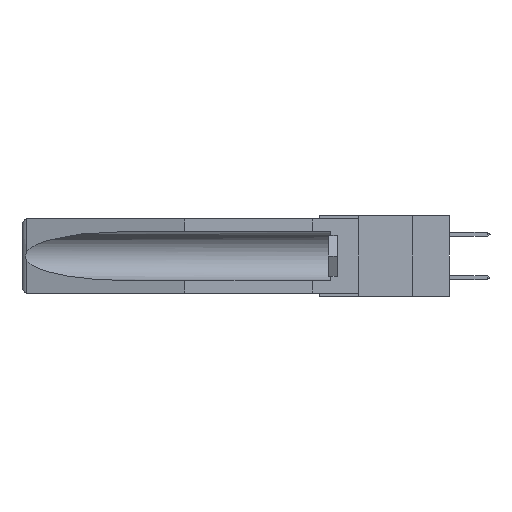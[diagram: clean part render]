
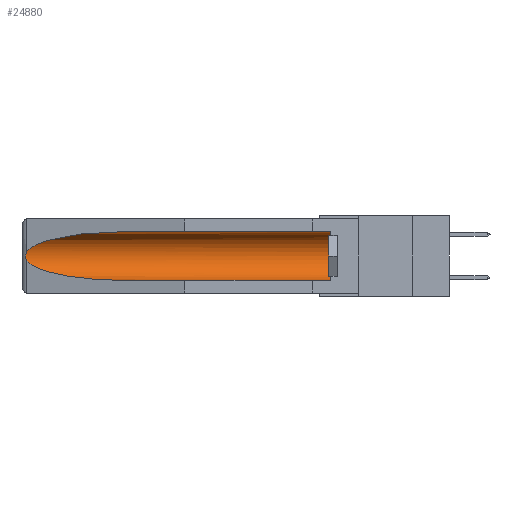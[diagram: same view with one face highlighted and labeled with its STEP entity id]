
A CAD part, left-side view. The second image highlights one B-rep face of the part: STEP entity #24880.
In plain terms, the highlighted cylindrical face has radius 2.857 mm (diameter 5.715 mm), a partial arc.
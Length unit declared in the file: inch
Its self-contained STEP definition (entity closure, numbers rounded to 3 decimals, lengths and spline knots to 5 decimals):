
#214 = DIRECTION ( 'NONE',  ( 0., 1., 0. ) ) ;
#863 = CARTESIAN_POINT ( 'NONE',  ( 0.26537, 1.52718, -0.19328 ) ) ;
#1735 = AXIS2_PLACEMENT_3D ( 'NONE', #17548, #19934, #3326 ) ;
#1859 = EDGE_CURVE ( 'NONE', #19956, #7978, #10673, .T. ) ;
#3016 = CARTESIAN_POINT ( 'NONE',  ( 0.155, 1.07973, -0.059 ) ) ;
#3326 = DIRECTION ( 'NONE',  ( 0., 0., 1. ) ) ;
#3481 = CARTESIAN_POINT ( 'NONE',  ( 0.26537, 1.52718, -0.14972 ) ) ;
#3606 =( BOUNDED_CURVE ( )  B_SPLINE_CURVE ( 3, ( #11257, #11065, #22783, #15631 ),
 .UNSPECIFIED., .F., .F. ) 
 B_SPLINE_CURVE_WITH_KNOTS ( ( 4, 4 ),
 ( 0.1948, 1.5708 ),
 .UNSPECIFIED. ) 
 CURVE ( )  GEOMETRIC_REPRESENTATION_ITEM ( )  RATIONAL_B_SPLINE_CURVE ( ( 1., 0.848, 0.848, 1. ) ) 
 REPRESENTATION_ITEM ( '' )  );
#3780 = EDGE_CURVE ( 'NONE', #7156, #20496, #21490, .T. ) ;
#5236 = EDGE_LOOP ( 'NONE', ( #13361, #5335, #15770, #25116, #20917, #25081 ) ) ;
#5335 = ORIENTED_EDGE ( 'NONE', *, *, #9148, .T. ) ;
#6289 = CARTESIAN_POINT ( 'NONE',  ( 0.2675, 1.53308, -0.17534 ) ) ;
#7156 = VERTEX_POINT ( 'NONE', #22638 ) ;
#7978 = VERTEX_POINT ( 'NONE', #10815 ) ;
#8559 = CARTESIAN_POINT ( 'NONE',  ( 0.26537, 1.52718, -0.14972 ) ) ;
#8656 = CARTESIAN_POINT ( 'NONE',  ( 0.2673, 1.5327, -0.16383 ) ) ;
#9148 = EDGE_CURVE ( 'NONE', #20496, #27413, #15591, .T. ) ;
#9600 = VERTEX_POINT ( 'NONE', #24937 ) ;
#10149 = CARTESIAN_POINT ( 'NONE',  ( 0.155, -0.30754, -0.1715 ) ) ;
#10673 = CIRCLE ( 'NONE', #1735, 0.1125 ) ;
#10815 = CARTESIAN_POINT ( 'NONE',  ( 0.155, 0.126, -0.059 ) ) ;
#11011 = CARTESIAN_POINT ( 'NONE',  ( 0.26537, 1.52718, -0.19328 ) ) ;
#11060 = CARTESIAN_POINT ( 'NONE',  ( 0.26597, 1.5296, -0.19026 ) ) ;
#11065 = CARTESIAN_POINT ( 'NONE',  ( 0.25451, 1.48313, -0.24835 ) ) ;
#11257 = CARTESIAN_POINT ( 'NONE',  ( 0.26537, 1.52718, -0.19328 ) ) ;
#13358 = CARTESIAN_POINT ( 'NONE',  ( 0.26654, 1.53092, -0.15636 ) ) ;
#13361 = ORIENTED_EDGE ( 'NONE', *, *, #3780, .T. ) ;
#14021 = DIRECTION ( 'NONE',  ( 0., 1., 0. ) ) ;
#14847 = LINE ( 'NONE', #25965, #16313 ) ;
#15588 = CARTESIAN_POINT ( 'NONE',  ( 0.155, 0.126, -0.284 ) ) ;
#15591 = B_SPLINE_CURVE_WITH_KNOTS ( 'NONE', 3,
 ( #8559, #27561, #13358, #8656, #18232, #6289, #24556, #26954, #11060, #863 ),
 .UNSPECIFIED., .F., .F.,
 ( 4, 2, 2, 2, 4 ),
 ( 0., 0.00029, 0.00058, 0.00087, 0.00117 ),
 .UNSPECIFIED. ) ;
#15631 = CARTESIAN_POINT ( 'NONE',  ( 0.155, 1.07973, -0.284 ) ) ;
#15770 = ORIENTED_EDGE ( 'NONE', *, *, #29196, .T. ) ;
#16313 = VECTOR ( 'NONE', #14021, 39.37008 ) ;
#16594 = AXIS2_PLACEMENT_3D ( 'NONE', #10149, #21783, #21884 ) ;
#17254 = CARTESIAN_POINT ( 'NONE',  ( 0.25451, 1.48313, -0.09465 ) ) ;
#17548 = CARTESIAN_POINT ( 'NONE',  ( 0.155, 0.126, -0.1715 ) ) ;
#18232 = CARTESIAN_POINT ( 'NONE',  ( 0.2675, 1.53308, -0.16763 ) ) ;
#18387 = LINE ( 'NONE', #23995, #26942 ) ;
#19660 = EDGE_CURVE ( 'NONE', #19956, #9600, #14847, .T. ) ;
#19934 = DIRECTION ( 'NONE',  ( 0., -1., 0. ) ) ;
#19956 = VERTEX_POINT ( 'NONE', #15588 ) ;
#20496 = VERTEX_POINT ( 'NONE', #3481 ) ;
#20579 = CYLINDRICAL_SURFACE ( 'NONE', #16594, 0.1125 ) ;
#20917 = ORIENTED_EDGE ( 'NONE', *, *, #1859, .T. ) ;
#21490 =( BOUNDED_CURVE ( )  B_SPLINE_CURVE ( 3, ( #3016, #28868, #17254, #26721 ),
 .UNSPECIFIED., .F., .F. ) 
 B_SPLINE_CURVE_WITH_KNOTS ( ( 4, 4 ),
 ( 4.71239, 6.08839 ),
 .UNSPECIFIED. ) 
 CURVE ( )  GEOMETRIC_REPRESENTATION_ITEM ( )  RATIONAL_B_SPLINE_CURVE ( ( 1., 0.848, 0.848, 1. ) ) 
 REPRESENTATION_ITEM ( '' )  );
#21783 = DIRECTION ( 'NONE',  ( 0., 1., 0. ) ) ;
#21884 = DIRECTION ( 'NONE',  ( 0., 0., 1. ) ) ;
#21915 = EDGE_CURVE ( 'NONE', #7978, #7156, #18387, .T. ) ;
#22638 = CARTESIAN_POINT ( 'NONE',  ( 0.155, 1.07973, -0.059 ) ) ;
#22783 = CARTESIAN_POINT ( 'NONE',  ( 0.21114, 1.30732, -0.284 ) ) ;
#23995 = CARTESIAN_POINT ( 'NONE',  ( 0.155, -0.30754, -0.059 ) ) ;
#24556 = CARTESIAN_POINT ( 'NONE',  ( 0.2673, 1.53269, -0.17917 ) ) ;
#24880 = ADVANCED_FACE ( 'NONE', ( #28349 ), #20579, .F. ) ;
#24937 = CARTESIAN_POINT ( 'NONE',  ( 0.155, 1.07973, -0.284 ) ) ;
#25081 = ORIENTED_EDGE ( 'NONE', *, *, #21915, .T. ) ;
#25116 = ORIENTED_EDGE ( 'NONE', *, *, #19660, .F. ) ;
#25965 = CARTESIAN_POINT ( 'NONE',  ( 0.155, -0.30754, -0.284 ) ) ;
#26721 = CARTESIAN_POINT ( 'NONE',  ( 0.26537, 1.52718, -0.14972 ) ) ;
#26942 = VECTOR ( 'NONE', #214, 39.37008 ) ;
#26954 = CARTESIAN_POINT ( 'NONE',  ( 0.26655, 1.53094, -0.18657 ) ) ;
#27413 = VERTEX_POINT ( 'NONE', #11011 ) ;
#27561 = CARTESIAN_POINT ( 'NONE',  ( 0.26597, 1.52961, -0.15275 ) ) ;
#28349 = FACE_OUTER_BOUND ( 'NONE', #5236, .T. ) ;
#28868 = CARTESIAN_POINT ( 'NONE',  ( 0.21114, 1.30732, -0.059 ) ) ;
#29196 = EDGE_CURVE ( 'NONE', #27413, #9600, #3606, .T. ) ;
